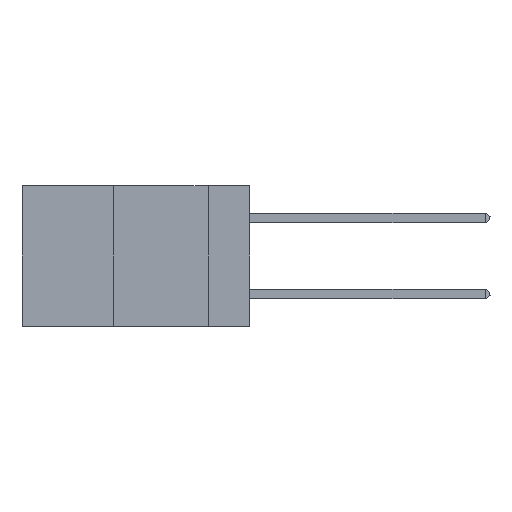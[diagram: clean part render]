
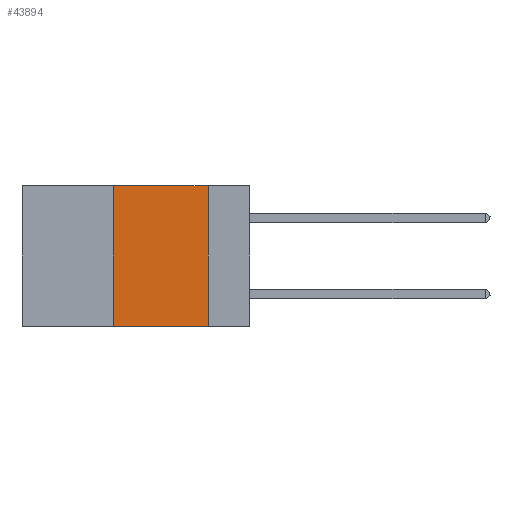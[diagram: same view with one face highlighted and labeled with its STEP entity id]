
A CAD part, left-side view. The second image highlights one B-rep face of the part: STEP entity #43894.
In plain terms, the highlighted planar face has unit normal (-1, 0, 0).
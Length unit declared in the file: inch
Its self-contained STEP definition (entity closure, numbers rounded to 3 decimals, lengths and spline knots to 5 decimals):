
#91 = VERTEX_POINT ( 'NONE', #38129 ) ;
#790 = LINE ( 'NONE', #45617, #4197 ) ;
#1482 = DIRECTION ( 'NONE',  ( 0., -1., 0. ) ) ;
#2949 = ORIENTED_EDGE ( 'NONE', *, *, #4620, .F. ) ;
#3923 = EDGE_CURVE ( 'NONE', #36567, #34449, #19044, .T. ) ;
#4197 = VECTOR ( 'NONE', #34655, 39.37008 ) ;
#4620 = EDGE_CURVE ( 'NONE', #34449, #10816, #790, .T. ) ;
#4666 = CARTESIAN_POINT ( 'NONE',  ( 0., 0.11, -0.37 ) ) ;
#6214 = CARTESIAN_POINT ( 'NONE',  ( 0., 0.6, -0.37 ) ) ;
#7943 = CARTESIAN_POINT ( 'NONE',  ( 0., 0.36, 0. ) ) ;
#9280 = ORIENTED_EDGE ( 'NONE', *, *, #19522, .T. ) ;
#10816 = VERTEX_POINT ( 'NONE', #4666 ) ;
#11445 = LINE ( 'NONE', #40654, #17108 ) ;
#11948 = AXIS2_PLACEMENT_3D ( 'NONE', #32495, #28680, #46400 ) ;
#12136 = EDGE_LOOP ( 'NONE', ( #2949, #42758, #37305, #9280 ) ) ;
#14556 = CARTESIAN_POINT ( 'NONE',  ( 0., 0.11, 0. ) ) ;
#17108 = VECTOR ( 'NONE', #22495, 39.37008 ) ;
#19044 = LINE ( 'NONE', #23147, #34858 ) ;
#19522 = EDGE_CURVE ( 'NONE', #91, #10816, #37050, .T. ) ;
#22495 = DIRECTION ( 'NONE',  ( 0., 0., 1. ) ) ;
#23147 = CARTESIAN_POINT ( 'NONE',  ( 0., 0.6, 0. ) ) ;
#23317 = FACE_OUTER_BOUND ( 'NONE', #12136, .T. ) ;
#28680 = DIRECTION ( 'NONE',  ( 1., 0., 0. ) ) ;
#32495 = CARTESIAN_POINT ( 'NONE',  ( 0., 0.6, 0. ) ) ;
#34449 = VERTEX_POINT ( 'NONE', #14556 ) ;
#34655 = DIRECTION ( 'NONE',  ( 0., 0., -1. ) ) ;
#34858 = VECTOR ( 'NONE', #1482, 39.37008 ) ;
#35496 = PLANE ( 'NONE',  #11948 ) ;
#36567 = VERTEX_POINT ( 'NONE', #7943 ) ;
#37050 = LINE ( 'NONE', #6214, #44878 ) ;
#37305 = ORIENTED_EDGE ( 'NONE', *, *, #44171, .F. ) ;
#38129 = CARTESIAN_POINT ( 'NONE',  ( 0., 0.36, -0.37 ) ) ;
#38478 = DIRECTION ( 'NONE',  ( 0., -1., 0. ) ) ;
#40654 = CARTESIAN_POINT ( 'NONE',  ( 0., 0.36, 0. ) ) ;
#42758 = ORIENTED_EDGE ( 'NONE', *, *, #3923, .F. ) ;
#43894 = ADVANCED_FACE ( 'NONE', ( #23317 ), #35496, .F. ) ;
#44171 = EDGE_CURVE ( 'NONE', #91, #36567, #11445, .T. ) ;
#44878 = VECTOR ( 'NONE', #38478, 39.37008 ) ;
#45617 = CARTESIAN_POINT ( 'NONE',  ( 0., 0.11, 0. ) ) ;
#46400 = DIRECTION ( 'NONE',  ( 0., 0., -1. ) ) ;
